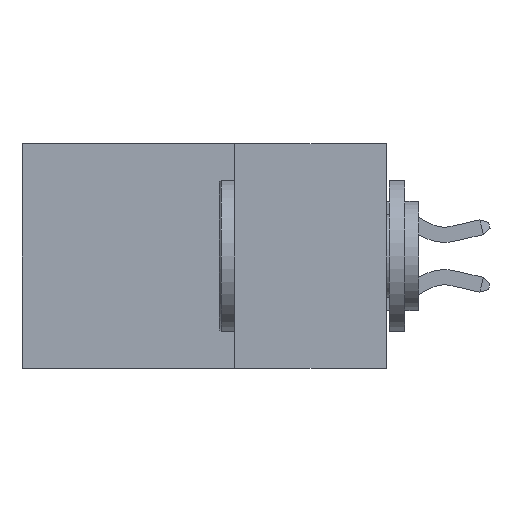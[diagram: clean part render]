
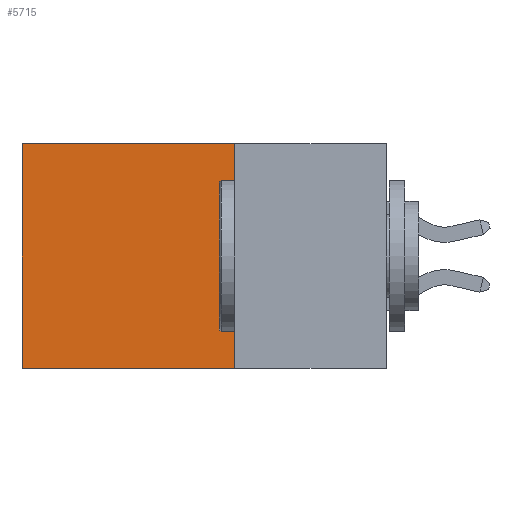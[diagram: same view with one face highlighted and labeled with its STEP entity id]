
A CAD part, left-side view. The second image highlights one B-rep face of the part: STEP entity #5715.
In plain terms, the highlighted planar face has unit normal (-1, 0, 0).
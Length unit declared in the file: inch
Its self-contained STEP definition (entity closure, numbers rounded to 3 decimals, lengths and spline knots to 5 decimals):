
#269 = CARTESIAN_POINT ( 'NONE',  ( 0.2615, 0.6, -0.37 ) ) ;
#1798 = VERTEX_POINT ( 'NONE', #18436 ) ;
#3047 = ORIENTED_EDGE ( 'NONE', *, *, #5282, .T. ) ;
#4562 = AXIS2_PLACEMENT_3D ( 'NONE', #13583, #15879, #24393 ) ;
#4844 = VECTOR ( 'NONE', #12095, 39.37008 ) ;
#5282 = EDGE_CURVE ( 'NONE', #1798, #26672, #13088, .T. ) ;
#5715 = ADVANCED_FACE ( 'NONE', ( #22495 ), #15600, .F. ) ;
#5763 = LINE ( 'NONE', #7933, #4844 ) ;
#5933 = ORIENTED_EDGE ( 'NONE', *, *, #18407, .T. ) ;
#5993 = VECTOR ( 'NONE', #28176, 39.37008 ) ;
#6550 = VERTEX_POINT ( 'NONE', #23458 ) ;
#7395 = DIRECTION ( 'NONE',  ( 0., 0., -1. ) ) ;
#7819 = VECTOR ( 'NONE', #7395, 39.37008 ) ;
#7933 = CARTESIAN_POINT ( 'NONE',  ( 0.2615, 0.25, 0. ) ) ;
#8205 = EDGE_CURVE ( 'NONE', #6550, #25217, #16161, .T. ) ;
#10150 = EDGE_LOOP ( 'NONE', ( #3047, #27430, #23977, #5933 ) ) ;
#10929 = DIRECTION ( 'NONE',  ( 0., 0., -1. ) ) ;
#12095 = DIRECTION ( 'NONE',  ( 0., 1., 0. ) ) ;
#12255 = VECTOR ( 'NONE', #10929, 39.37008 ) ;
#13041 = LINE ( 'NONE', #15335, #5993 ) ;
#13088 = LINE ( 'NONE', #269, #12255 ) ;
#13583 = CARTESIAN_POINT ( 'NONE',  ( 0.2615, 0.25, -0.37 ) ) ;
#13728 = CARTESIAN_POINT ( 'NONE',  ( 0.2615, 0.25, -0.37 ) ) ;
#15335 = CARTESIAN_POINT ( 'NONE',  ( 0.2615, 0.25, -0.37 ) ) ;
#15600 = PLANE ( 'NONE',  #4562 ) ;
#15879 = DIRECTION ( 'NONE',  ( 1., 0., 0. ) ) ;
#16161 = LINE ( 'NONE', #22934, #7819 ) ;
#18407 = EDGE_CURVE ( 'NONE', #6550, #1798, #5763, .T. ) ;
#18436 = CARTESIAN_POINT ( 'NONE',  ( 0.2615, 0.6, 0. ) ) ;
#21078 = CARTESIAN_POINT ( 'NONE',  ( 0.2615, 0.6, -0.37 ) ) ;
#22495 = FACE_OUTER_BOUND ( 'NONE', #10150, .T. ) ;
#22934 = CARTESIAN_POINT ( 'NONE',  ( 0.2615, 0.25, -0.37 ) ) ;
#23458 = CARTESIAN_POINT ( 'NONE',  ( 0.2615, 0.25, 0. ) ) ;
#23977 = ORIENTED_EDGE ( 'NONE', *, *, #8205, .F. ) ;
#24393 = DIRECTION ( 'NONE',  ( 0., 0., -1. ) ) ;
#24911 = EDGE_CURVE ( 'NONE', #25217, #26672, #13041, .T. ) ;
#25217 = VERTEX_POINT ( 'NONE', #13728 ) ;
#26672 = VERTEX_POINT ( 'NONE', #21078 ) ;
#27430 = ORIENTED_EDGE ( 'NONE', *, *, #24911, .F. ) ;
#28176 = DIRECTION ( 'NONE',  ( 0., 1., 0. ) ) ;
